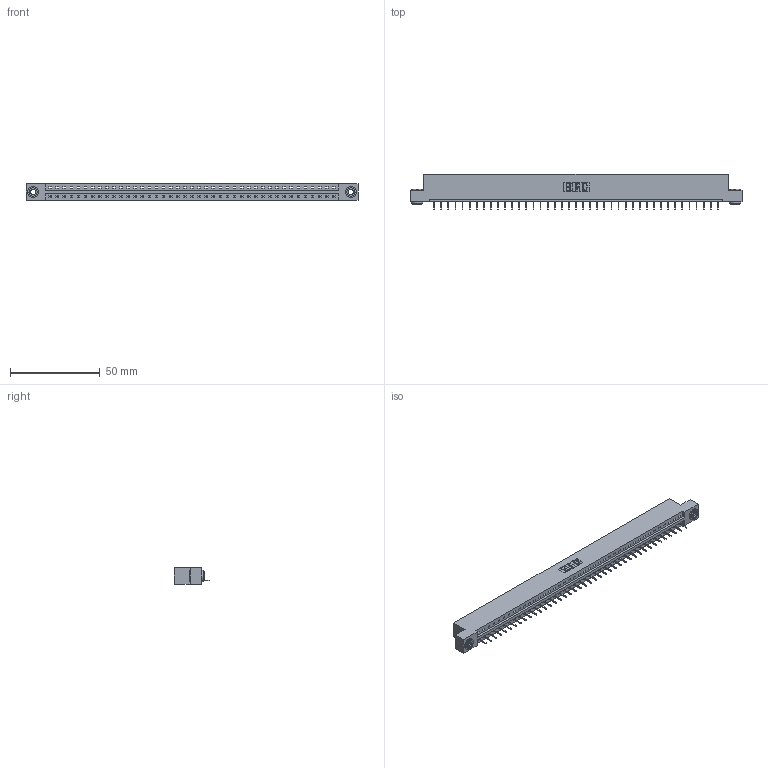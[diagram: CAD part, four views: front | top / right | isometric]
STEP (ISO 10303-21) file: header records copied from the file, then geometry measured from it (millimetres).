
FILE_DESCRIPTION (( 'STEP AP203' ), '1' );
FILE_NAME ('387-041-524-103.STEP', '2019-10-04T19:39:30', ( '' ), ( '' ), 'SwSTEP 2.0', 'SolidWorks 2016', '' );
FILE_SCHEMA (( 'CONFIG_CONTROL_DESIGN' ));
Length unit declared in the file: inch
Products named in the file (4): 337 Part_Flush Mounting Lugs - 0.156 Dia-TH; 345-250-002_345-250-002-102; 345-292-001_345-293-124; 387-041-524-103
Assembly tree (44 placements, depth 2):
  387-041-524-103
    337 Part_Flush Mounting Lugs - 0.156 Dia-TH
    345-292-001_345-293-124  x41
    345-250-002_345-250-002-102  x2
Bounding box: 185.47 x 19.69 x 9.4 mm (x, y, z)
Volume: 19121.5 mm3; surface area: 19416.8 mm2
Topology: 44 solids, 44 shells, 2858 faces, 8259 edges, 5338 vertices
Faces by surface type: plane 2212, cylinder 638, cone 8
Entity records: 31330 total; most frequent: CARTESIAN_POINT 5432, ORIENTED_EDGE 5402, DIRECTION 4609, EDGE_CURVE 2701, LINE 2553, VECTOR 2553, VERTEX_POINT 1794, AXIS2_PLACEMENT_3D 1028
